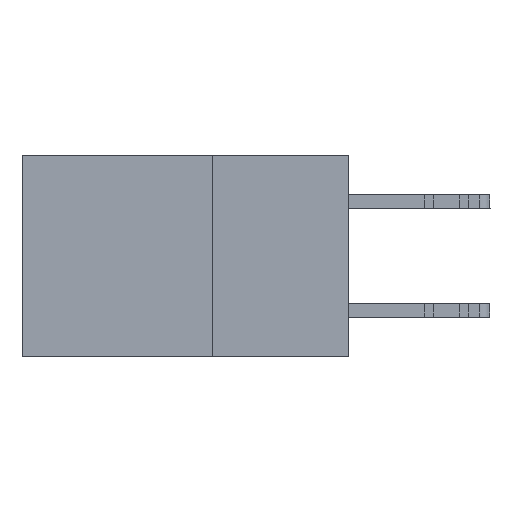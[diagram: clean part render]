
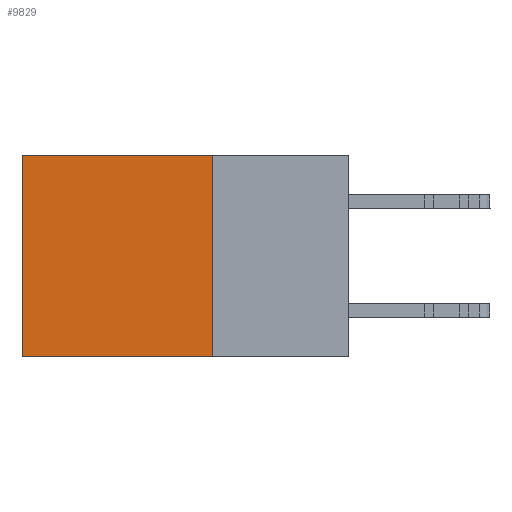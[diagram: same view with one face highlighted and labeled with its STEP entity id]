
A CAD part, left-side view. The second image highlights one B-rep face of the part: STEP entity #9829.
In plain terms, the highlighted planar face has unit normal (-1, 0, 0).
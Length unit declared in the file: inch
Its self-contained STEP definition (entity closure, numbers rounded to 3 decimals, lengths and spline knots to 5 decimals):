
#667 = VERTEX_POINT ( 'NONE', #21279 ) ;
#964 = DIRECTION ( 'NONE',  ( 1., 0., 0. ) ) ;
#1741 = CARTESIAN_POINT ( 'NONE',  ( 0.2615, 0.25, 0. ) ) ;
#2163 = LINE ( 'NONE', #11516, #20476 ) ;
#2931 = ORIENTED_EDGE ( 'NONE', *, *, #14172, .F. ) ;
#2988 = DIRECTION ( 'NONE',  ( 0., 0., -1. ) ) ;
#3408 = EDGE_LOOP ( 'NONE', ( #20414, #13757, #2931, #12371 ) ) ;
#4305 = EDGE_CURVE ( 'NONE', #14407, #18388, #6848, .T. ) ;
#5050 = LINE ( 'NONE', #16170, #6802 ) ;
#5962 = CARTESIAN_POINT ( 'NONE',  ( 0.2615, 0.6, -0.37 ) ) ;
#6528 = DIRECTION ( 'NONE',  ( 0., 0., -1. ) ) ;
#6651 = CARTESIAN_POINT ( 'NONE',  ( 0.2615, 0.25, -0.37 ) ) ;
#6802 = VECTOR ( 'NONE', #2988, 39.37008 ) ;
#6848 = LINE ( 'NONE', #16033, #18151 ) ;
#8408 = AXIS2_PLACEMENT_3D ( 'NONE', #15857, #964, #19347 ) ;
#8950 = EDGE_CURVE ( 'NONE', #667, #18388, #5050, .T. ) ;
#9829 = ADVANCED_FACE ( 'NONE', ( #17320 ), #12125, .F. ) ;
#11516 = CARTESIAN_POINT ( 'NONE',  ( 0.2615, 0.25, 0. ) ) ;
#12125 = PLANE ( 'NONE',  #8408 ) ;
#12371 = ORIENTED_EDGE ( 'NONE', *, *, #21618, .T. ) ;
#13136 = CARTESIAN_POINT ( 'NONE',  ( 0.2615, 0.25, -0.37 ) ) ;
#13648 = VECTOR ( 'NONE', #6528, 39.37008 ) ;
#13684 = DIRECTION ( 'NONE',  ( 0., 1., 0. ) ) ;
#13757 = ORIENTED_EDGE ( 'NONE', *, *, #4305, .F. ) ;
#13857 = DIRECTION ( 'NONE',  ( 0., 1., 0. ) ) ;
#14172 = EDGE_CURVE ( 'NONE', #16205, #14407, #22828, .T. ) ;
#14407 = VERTEX_POINT ( 'NONE', #13136 ) ;
#15857 = CARTESIAN_POINT ( 'NONE',  ( 0.2615, 0.25, -0.37 ) ) ;
#16033 = CARTESIAN_POINT ( 'NONE',  ( 0.2615, 0.25, -0.37 ) ) ;
#16170 = CARTESIAN_POINT ( 'NONE',  ( 0.2615, 0.6, -0.37 ) ) ;
#16205 = VERTEX_POINT ( 'NONE', #1741 ) ;
#17320 = FACE_OUTER_BOUND ( 'NONE', #3408, .T. ) ;
#18151 = VECTOR ( 'NONE', #13857, 39.37008 ) ;
#18388 = VERTEX_POINT ( 'NONE', #5962 ) ;
#19347 = DIRECTION ( 'NONE',  ( 0., 0., -1. ) ) ;
#20414 = ORIENTED_EDGE ( 'NONE', *, *, #8950, .T. ) ;
#20476 = VECTOR ( 'NONE', #13684, 39.37008 ) ;
#21279 = CARTESIAN_POINT ( 'NONE',  ( 0.2615, 0.6, 0. ) ) ;
#21618 = EDGE_CURVE ( 'NONE', #16205, #667, #2163, .T. ) ;
#22828 = LINE ( 'NONE', #6651, #13648 ) ;
